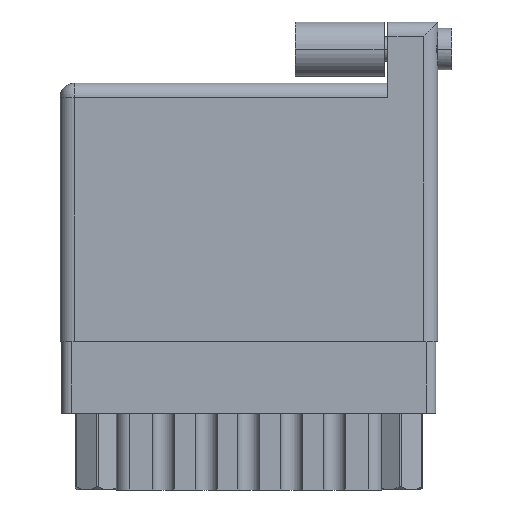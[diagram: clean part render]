
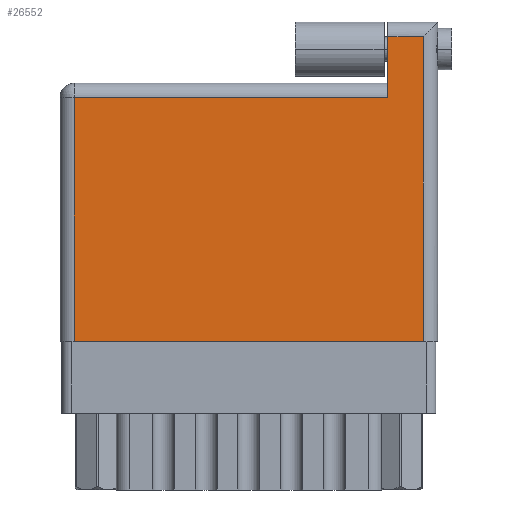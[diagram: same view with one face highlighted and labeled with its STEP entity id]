
A CAD part, front view. The second image highlights one B-rep face of the part: STEP entity #26552.
In plain terms, the highlighted face is planar.
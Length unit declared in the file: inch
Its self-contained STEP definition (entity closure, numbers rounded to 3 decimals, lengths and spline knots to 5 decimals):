
#365 = VERTEX_POINT ( 'NONE', #2923 ) ;
#1916 = VERTEX_POINT ( 'NONE', #20598 ) ;
#2923 = CARTESIAN_POINT ( 'NONE',  ( 1.275, 0., 0. ) ) ;
#3360 = EDGE_CURVE ( 'NONE', #6479, #365, #10655, .T. ) ;
#3447 = LINE ( 'NONE', #24867, #34315 ) ;
#3459 = DIRECTION ( 'NONE',  ( -1., 0., 0. ) ) ;
#4783 = EDGE_CURVE ( 'NONE', #1916, #6479, #23297, .T. ) ;
#5740 = CARTESIAN_POINT ( 'NONE',  ( 0., 0., 0. ) ) ;
#6450 = LINE ( 'NONE', #29860, #20154 ) ;
#6479 = VERTEX_POINT ( 'NONE', #12081 ) ;
#6624 = CARTESIAN_POINT ( 'NONE',  ( 0.05, 0., 0. ) ) ;
#7482 = VERTEX_POINT ( 'NONE', #15690 ) ;
#8033 = DIRECTION ( 'NONE',  ( 1., 0., 0. ) ) ;
#9185 = EDGE_LOOP ( 'NONE', ( #28344, #33101, #20323, #21429, #9889, #31136 ) ) ;
#9889 = ORIENTED_EDGE ( 'NONE', *, *, #31593, .T. ) ;
#10109 = DIRECTION ( 'NONE',  ( -1., 0., 0. ) ) ;
#10135 = DIRECTION ( 'NONE',  ( 0., 0., -1. ) ) ;
#10655 = LINE ( 'NONE', #5740, #25525 ) ;
#10832 = FACE_OUTER_BOUND ( 'NONE', #9185, .T. ) ;
#10836 = VECTOR ( 'NONE', #23119, 39.37008 ) ;
#12081 = CARTESIAN_POINT ( 'NONE',  ( 0.05, 0., 0. ) ) ;
#12231 = VERTEX_POINT ( 'NONE', #27195 ) ;
#12828 = EDGE_CURVE ( 'NONE', #12231, #7482, #19427, .T. ) ;
#15301 = VECTOR ( 'NONE', #3459, 39.37008 ) ;
#15363 = VECTOR ( 'NONE', #10109, 39.37008 ) ;
#15690 = CARTESIAN_POINT ( 'NONE',  ( 1.15, 1.07, 0. ) ) ;
#16518 = DIRECTION ( 'NONE',  ( 0., 1., 0. ) ) ;
#16784 = EDGE_CURVE ( 'NONE', #365, #12231, #6450, .T. ) ;
#19427 = LINE ( 'NONE', #33133, #15301 ) ;
#20154 = VECTOR ( 'NONE', #16518, 39.37008 ) ;
#20323 = ORIENTED_EDGE ( 'NONE', *, *, #12828, .T. ) ;
#20598 = CARTESIAN_POINT ( 'NONE',  ( 0.05, 0.856, 0. ) ) ;
#20859 = DIRECTION ( 'NONE',  ( -1., 0., 0. ) ) ;
#21429 = ORIENTED_EDGE ( 'NONE', *, *, #28523, .T. ) ;
#21544 = CARTESIAN_POINT ( 'NONE',  ( 0., 0.906, 0. ) ) ;
#23119 = DIRECTION ( 'NONE',  ( 0., -1., 0. ) ) ;
#23297 = LINE ( 'NONE', #6624, #10836 ) ;
#23298 = CARTESIAN_POINT ( 'NONE',  ( 0., 0.856, 0. ) ) ;
#23532 = CARTESIAN_POINT ( 'NONE',  ( 1.15, 0.856, 0. ) ) ;
#24066 = AXIS2_PLACEMENT_3D ( 'NONE', #21544, #10135, #20859 ) ;
#24867 = CARTESIAN_POINT ( 'NONE',  ( 1.15, 1.12, 0. ) ) ;
#25204 = DIRECTION ( 'NONE',  ( 0., -1., 0. ) ) ;
#25525 = VECTOR ( 'NONE', #8033, 39.37008 ) ;
#26552 = ADVANCED_FACE ( 'NONE', ( #10832 ), #31569, .F. ) ;
#27195 = CARTESIAN_POINT ( 'NONE',  ( 1.275, 1.07, 0. ) ) ;
#28344 = ORIENTED_EDGE ( 'NONE', *, *, #3360, .T. ) ;
#28523 = EDGE_CURVE ( 'NONE', #7482, #32543, #3447, .T. ) ;
#29860 = CARTESIAN_POINT ( 'NONE',  ( 1.275, 1.12, 0. ) ) ;
#31136 = ORIENTED_EDGE ( 'NONE', *, *, #4783, .T. ) ;
#31547 = LINE ( 'NONE', #23298, #15363 ) ;
#31569 = PLANE ( 'NONE',  #24066 ) ;
#31593 = EDGE_CURVE ( 'NONE', #32543, #1916, #31547, .T. ) ;
#32543 = VERTEX_POINT ( 'NONE', #23532 ) ;
#33101 = ORIENTED_EDGE ( 'NONE', *, *, #16784, .T. ) ;
#33133 = CARTESIAN_POINT ( 'NONE',  ( 0., 1.07, 0. ) ) ;
#34315 = VECTOR ( 'NONE', #25204, 39.37008 ) ;
